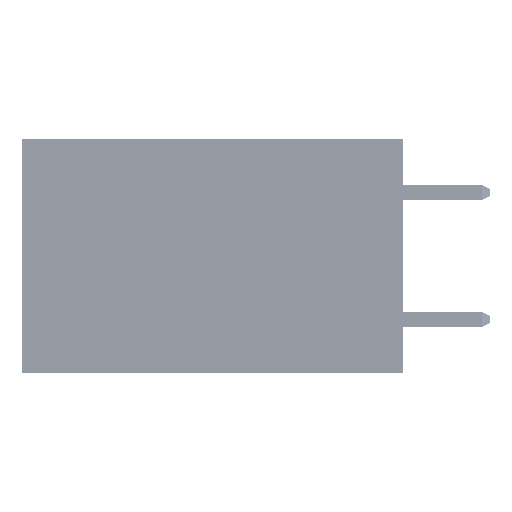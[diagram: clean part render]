
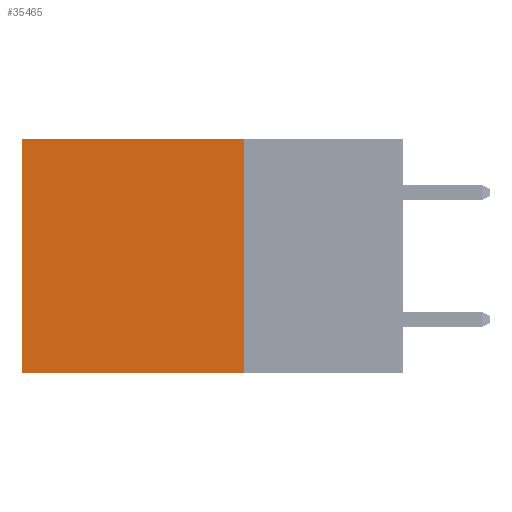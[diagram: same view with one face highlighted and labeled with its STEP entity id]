
A CAD part, left-side view. The second image highlights one B-rep face of the part: STEP entity #35465.
In plain terms, the highlighted planar face has unit normal (-1, 0, 0).
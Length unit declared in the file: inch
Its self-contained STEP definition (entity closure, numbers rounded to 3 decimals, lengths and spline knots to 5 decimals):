
#2801 = PLANE ( 'NONE',  #17466 ) ;
#2978 = VERTEX_POINT ( 'NONE', #33585 ) ;
#6784 = LINE ( 'NONE', #35858, #15573 ) ;
#9687 = EDGE_CURVE ( 'NONE', #38991, #2978, #44675, .T. ) ;
#13032 = ORIENTED_EDGE ( 'NONE', *, *, #42690, .T. ) ;
#13225 = DIRECTION ( 'NONE',  ( 0., 1., 0. ) ) ;
#13378 = DIRECTION ( 'NONE',  ( 0., 1., 0. ) ) ;
#15573 = VECTOR ( 'NONE', #13378, 39.37008 ) ;
#16790 = ORIENTED_EDGE ( 'NONE', *, *, #41862, .F. ) ;
#17181 = LINE ( 'NONE', #42931, #41243 ) ;
#17253 = CARTESIAN_POINT ( 'NONE',  ( 0.2875, 0.6, 0. ) ) ;
#17272 = DIRECTION ( 'NONE',  ( 0., 0., -1. ) ) ;
#17466 = AXIS2_PLACEMENT_3D ( 'NONE', #21167, #39042, #27751 ) ;
#17642 = VECTOR ( 'NONE', #17272, 39.37008 ) ;
#20470 = EDGE_CURVE ( 'NONE', #38991, #40362, #6784, .T. ) ;
#21167 = CARTESIAN_POINT ( 'NONE',  ( 0.2875, 0.25, 0. ) ) ;
#22314 = CARTESIAN_POINT ( 'NONE',  ( 0.2875, 0.6, -0.37 ) ) ;
#23535 = CARTESIAN_POINT ( 'NONE',  ( 0.2875, 0.25, 0. ) ) ;
#26999 = CARTESIAN_POINT ( 'NONE',  ( 0.2875, 0.6, 0. ) ) ;
#27751 = DIRECTION ( 'NONE',  ( 0., 0., -1. ) ) ;
#28827 = VECTOR ( 'NONE', #43031, 39.37008 ) ;
#29920 = EDGE_LOOP ( 'NONE', ( #13032, #16790, #35600, #35147 ) ) ;
#31634 = FACE_OUTER_BOUND ( 'NONE', #29920, .T. ) ;
#33585 = CARTESIAN_POINT ( 'NONE',  ( 0.2875, 0.25, -0.37 ) ) ;
#35147 = ORIENTED_EDGE ( 'NONE', *, *, #20470, .T. ) ;
#35465 = ADVANCED_FACE ( 'NONE', ( #31634 ), #2801, .F. ) ;
#35600 = ORIENTED_EDGE ( 'NONE', *, *, #9687, .F. ) ;
#35858 = CARTESIAN_POINT ( 'NONE',  ( 0.2875, 0.25, 0. ) ) ;
#38991 = VERTEX_POINT ( 'NONE', #45417 ) ;
#39042 = DIRECTION ( 'NONE',  ( 1., 0., 0. ) ) ;
#40362 = VERTEX_POINT ( 'NONE', #26999 ) ;
#41243 = VECTOR ( 'NONE', #13225, 39.37008 ) ;
#41862 = EDGE_CURVE ( 'NONE', #2978, #43586, #17181, .T. ) ;
#42690 = EDGE_CURVE ( 'NONE', #40362, #43586, #45265, .T. ) ;
#42931 = CARTESIAN_POINT ( 'NONE',  ( 0.2875, 0.25, -0.37 ) ) ;
#43031 = DIRECTION ( 'NONE',  ( 0., 0., -1. ) ) ;
#43586 = VERTEX_POINT ( 'NONE', #22314 ) ;
#44675 = LINE ( 'NONE', #23535, #17642 ) ;
#45265 = LINE ( 'NONE', #17253, #28827 ) ;
#45417 = CARTESIAN_POINT ( 'NONE',  ( 0.2875, 0.25, 0. ) ) ;
